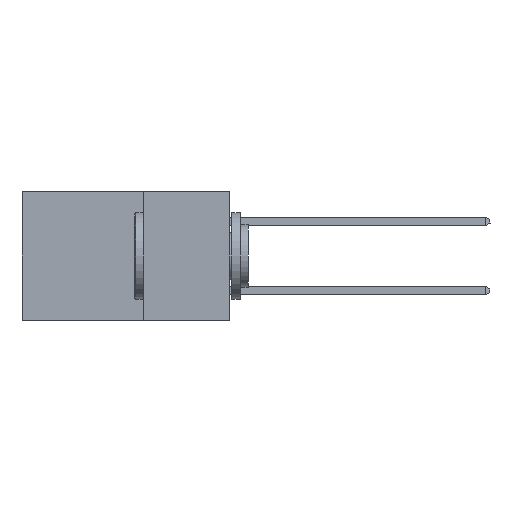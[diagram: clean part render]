
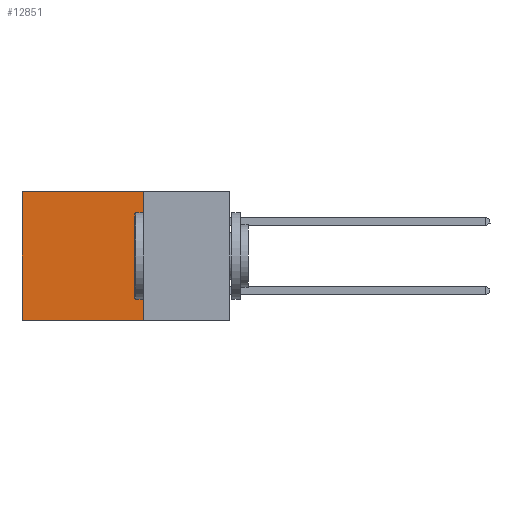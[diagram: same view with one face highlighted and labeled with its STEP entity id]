
A CAD part, left-side view. The second image highlights one B-rep face of the part: STEP entity #12851.
In plain terms, the highlighted planar face has unit normal (-1, 0, 0).
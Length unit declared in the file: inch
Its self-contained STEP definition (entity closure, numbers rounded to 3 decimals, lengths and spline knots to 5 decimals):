
#344 = DIRECTION ( 'NONE',  ( 0., 1., 0. ) ) ;
#1249 = EDGE_CURVE ( 'NONE', #31137, #26178, #21956, .T. ) ;
#4622 = CARTESIAN_POINT ( 'NONE',  ( 0.298, 0.6, -0.37 ) ) ;
#4732 = CARTESIAN_POINT ( 'NONE',  ( 0.298, 0.25, 0. ) ) ;
#6884 = ORIENTED_EDGE ( 'NONE', *, *, #14869, .F. ) ;
#7817 = EDGE_CURVE ( 'NONE', #26178, #19236, #32815, .T. ) ;
#11184 = DIRECTION ( 'NONE',  ( 0., 0., -1. ) ) ;
#12030 = ORIENTED_EDGE ( 'NONE', *, *, #1249, .T. ) ;
#12851 = ADVANCED_FACE ( 'NONE', ( #21727 ), #30646, .F. ) ;
#14237 = CARTESIAN_POINT ( 'NONE',  ( 0.298, 0.25, -0.37 ) ) ;
#14264 = CARTESIAN_POINT ( 'NONE',  ( 0.298, 0.25, 0. ) ) ;
#14869 = EDGE_CURVE ( 'NONE', #31137, #29540, #16281, .T. ) ;
#15233 = CARTESIAN_POINT ( 'NONE',  ( 0.298, 0.25, -0.37 ) ) ;
#15837 = AXIS2_PLACEMENT_3D ( 'NONE', #4732, #17832, #25589 ) ;
#16281 = LINE ( 'NONE', #19019, #32391 ) ;
#17544 = CARTESIAN_POINT ( 'NONE',  ( 0.298, 0.6, 0. ) ) ;
#17832 = DIRECTION ( 'NONE',  ( 1., 0., 0. ) ) ;
#18728 = VECTOR ( 'NONE', #24841, 39.37008 ) ;
#19019 = CARTESIAN_POINT ( 'NONE',  ( 0.298, 0.25, 0. ) ) ;
#19236 = VERTEX_POINT ( 'NONE', #4622 ) ;
#19751 = EDGE_LOOP ( 'NONE', ( #21837, #31936, #6884, #12030 ) ) ;
#21245 = VECTOR ( 'NONE', #344, 39.37008 ) ;
#21727 = FACE_OUTER_BOUND ( 'NONE', #19751, .T. ) ;
#21837 = ORIENTED_EDGE ( 'NONE', *, *, #7817, .T. ) ;
#21956 = LINE ( 'NONE', #14264, #18728 ) ;
#22264 = EDGE_CURVE ( 'NONE', #29540, #19236, #26827, .T. ) ;
#23752 = CARTESIAN_POINT ( 'NONE',  ( 0.298, 0.6, 0. ) ) ;
#24841 = DIRECTION ( 'NONE',  ( 0., 1., 0. ) ) ;
#25589 = DIRECTION ( 'NONE',  ( 0., 0., -1. ) ) ;
#26178 = VERTEX_POINT ( 'NONE', #17544 ) ;
#26233 = CARTESIAN_POINT ( 'NONE',  ( 0.298, 0.25, 0. ) ) ;
#26827 = LINE ( 'NONE', #15233, #21245 ) ;
#29540 = VERTEX_POINT ( 'NONE', #14237 ) ;
#30646 = PLANE ( 'NONE',  #15837 ) ;
#31137 = VERTEX_POINT ( 'NONE', #26233 ) ;
#31562 = DIRECTION ( 'NONE',  ( 0., 0., -1. ) ) ;
#31936 = ORIENTED_EDGE ( 'NONE', *, *, #22264, .F. ) ;
#32391 = VECTOR ( 'NONE', #11184, 39.37008 ) ;
#32815 = LINE ( 'NONE', #23752, #33187 ) ;
#33187 = VECTOR ( 'NONE', #31562, 39.37008 ) ;
